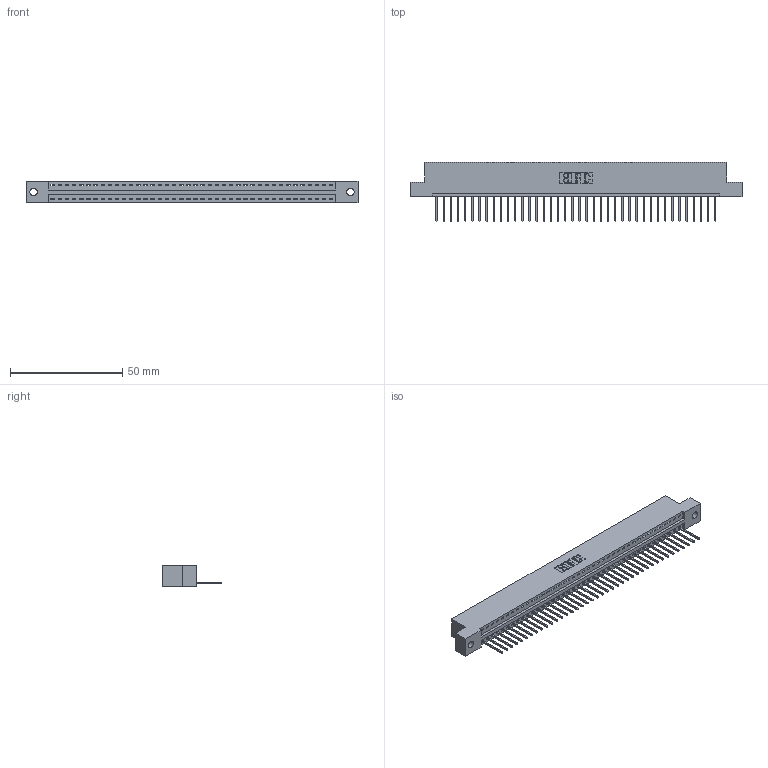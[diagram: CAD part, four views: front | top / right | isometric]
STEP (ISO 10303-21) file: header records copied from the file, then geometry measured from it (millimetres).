
FILE_DESCRIPTION (( 'STEP AP203' ), '1' );
FILE_NAME ('346-040-522-102.STEP', '2022-05-07T09:08:10', ( '' ), ( '' ), 'SwSTEP 2.0', 'SolidWorks 2020', '' );
FILE_SCHEMA (( 'CONFIG_CONTROL_DESIGN' ));
Length unit declared in the file: inch
Products named in the file (3): 346-040-522-102; 345-292-001_345-293-122; 346 Part_Flush Mounting Lugs - 0.128 Dia
Assembly tree (41 placements, depth 2):
  346-040-522-102
    346 Part_Flush Mounting Lugs - 0.128 Dia
    345-292-001_345-293-122  x40
Bounding box: 147.57 x 26.42 x 9.4 mm (x, y, z)
Volume: 14080.6 mm3; surface area: 17453.4 mm2
Topology: 41 solids, 41 shells, 2442 faces, 7369 edges, 4858 vertices
Faces by surface type: plane 1676, cylinder 766
Entity records: 25115 total; most frequent: CARTESIAN_POINT 4312, ORIENTED_EDGE 4286, DIRECTION 3807, EDGE_CURVE 2143, VECTOR 1851, LINE 1851, VERTEX_POINT 1426, AXIS2_PLACEMENT_3D 978
